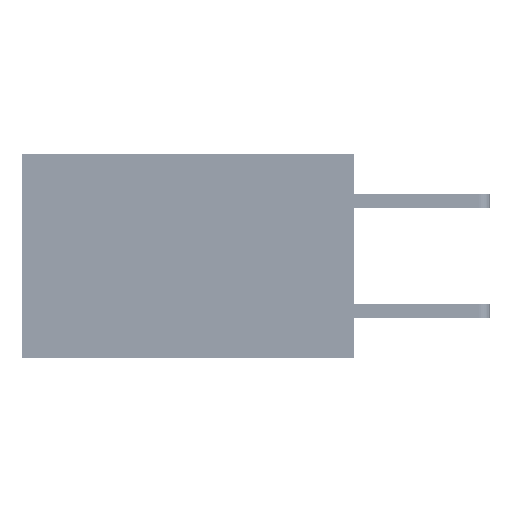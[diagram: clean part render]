
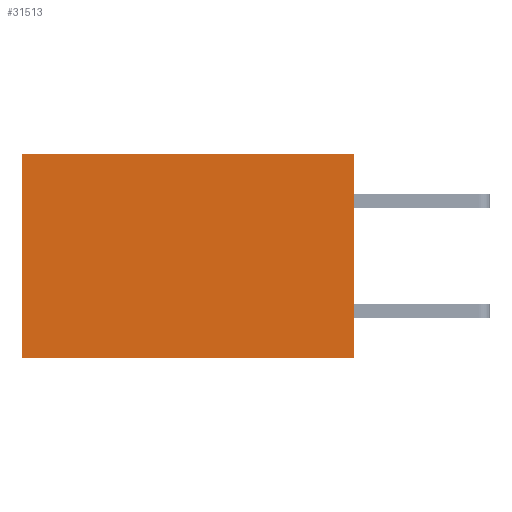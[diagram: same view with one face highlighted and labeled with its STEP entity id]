
A CAD part, left-side view. The second image highlights one B-rep face of the part: STEP entity #31513.
In plain terms, the highlighted planar face has unit normal (-1, 0, 0).
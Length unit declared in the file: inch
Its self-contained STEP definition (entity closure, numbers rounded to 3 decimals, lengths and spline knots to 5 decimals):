
#208 = VERTEX_POINT ( 'NONE', #39551 ) ;
#2305 = VERTEX_POINT ( 'NONE', #43509 ) ;
#3428 = DIRECTION ( 'NONE',  ( 0., 0., -1. ) ) ;
#5987 = VECTOR ( 'NONE', #36391, 39.37008 ) ;
#8308 = ORIENTED_EDGE ( 'NONE', *, *, #24685, .T. ) ;
#8354 = CARTESIAN_POINT ( 'NONE',  ( 0.2875, 0., -0.37 ) ) ;
#9535 = EDGE_LOOP ( 'NONE', ( #8308, #15114, #28470, #28936 ) ) ;
#13003 = DIRECTION ( 'NONE',  ( 0., 1., 0. ) ) ;
#13914 = EDGE_CURVE ( 'NONE', #41909, #2305, #31792, .T. ) ;
#15053 = LINE ( 'NONE', #15748, #5987 ) ;
#15114 = ORIENTED_EDGE ( 'NONE', *, *, #26948, .F. ) ;
#15184 = VECTOR ( 'NONE', #3428, 39.37008 ) ;
#15748 = CARTESIAN_POINT ( 'NONE',  ( 0.2875, 0., 0. ) ) ;
#15794 = AXIS2_PLACEMENT_3D ( 'NONE', #32065, #25061, #38977 ) ;
#16157 = EDGE_CURVE ( 'NONE', #41909, #27114, #15053, .T. ) ;
#16840 = FACE_OUTER_BOUND ( 'NONE', #9535, .T. ) ;
#18944 = LINE ( 'NONE', #23868, #15184 ) ;
#18946 = DIRECTION ( 'NONE',  ( 0., 1., 0. ) ) ;
#22947 = CARTESIAN_POINT ( 'NONE',  ( 0.2875, 0., -0.37 ) ) ;
#23868 = CARTESIAN_POINT ( 'NONE',  ( 0.2875, 0.6, 0. ) ) ;
#24685 = EDGE_CURVE ( 'NONE', #2305, #208, #18944, .T. ) ;
#25061 = DIRECTION ( 'NONE',  ( 1., 0., 0. ) ) ;
#26437 = VECTOR ( 'NONE', #13003, 39.37008 ) ;
#26948 = EDGE_CURVE ( 'NONE', #27114, #208, #34857, .T. ) ;
#27114 = VERTEX_POINT ( 'NONE', #22947 ) ;
#28470 = ORIENTED_EDGE ( 'NONE', *, *, #16157, .F. ) ;
#28936 = ORIENTED_EDGE ( 'NONE', *, *, #13914, .T. ) ;
#29725 = CARTESIAN_POINT ( 'NONE',  ( 0.2875, 0., 0. ) ) ;
#31091 = VECTOR ( 'NONE', #18946, 39.37008 ) ;
#31513 = ADVANCED_FACE ( 'NONE', ( #16840 ), #31904, .F. ) ;
#31792 = LINE ( 'NONE', #29725, #26437 ) ;
#31904 = PLANE ( 'NONE',  #15794 ) ;
#32065 = CARTESIAN_POINT ( 'NONE',  ( 0.2875, 0., 0. ) ) ;
#33693 = CARTESIAN_POINT ( 'NONE',  ( 0.2875, 0., 0. ) ) ;
#34857 = LINE ( 'NONE', #8354, #31091 ) ;
#36391 = DIRECTION ( 'NONE',  ( 0., 0., -1. ) ) ;
#38977 = DIRECTION ( 'NONE',  ( 0., 0., -1. ) ) ;
#39551 = CARTESIAN_POINT ( 'NONE',  ( 0.2875, 0.6, -0.37 ) ) ;
#41909 = VERTEX_POINT ( 'NONE', #33693 ) ;
#43509 = CARTESIAN_POINT ( 'NONE',  ( 0.2875, 0.6, 0. ) ) ;
